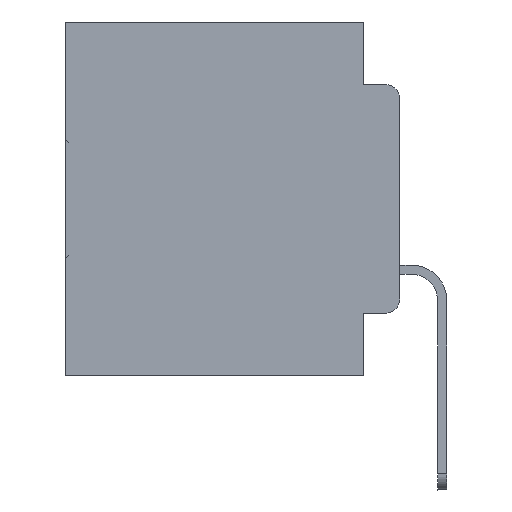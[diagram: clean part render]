
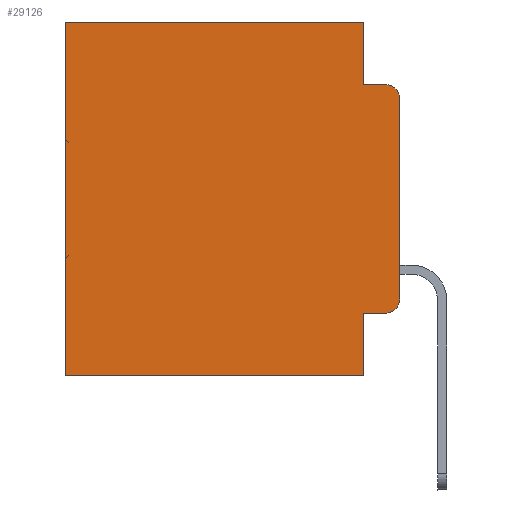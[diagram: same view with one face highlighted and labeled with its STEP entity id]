
A CAD part, left-side view. The second image highlights one B-rep face of the part: STEP entity #29126.
In plain terms, the highlighted planar face has unit normal (-1, 0, 0).
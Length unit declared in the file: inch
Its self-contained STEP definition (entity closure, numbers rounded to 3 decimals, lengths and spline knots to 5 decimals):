
#203 = ORIENTED_EDGE ( 'NONE', *, *, #19037, .F. ) ;
#785 = CARTESIAN_POINT ( 'NONE',  ( 0.298, 0.051, -0.4115 ) ) ;
#797 = CARTESIAN_POINT ( 'NONE',  ( 0.298, 0.051, -0.0885 ) ) ;
#1045 = CARTESIAN_POINT ( 'NONE',  ( 0.298, 0.051, -0.4115 ) ) ;
#1375 = LINE ( 'NONE', #26889, #33483 ) ;
#1922 = VERTEX_POINT ( 'NONE', #797 ) ;
#2664 = CARTESIAN_POINT ( 'NONE',  ( 0.298, 0.02, -0.0885 ) ) ;
#3745 = VECTOR ( 'NONE', #27782, 39.37008 ) ;
#3955 = CARTESIAN_POINT ( 'NONE',  ( 0.298, 0., 0. ) ) ;
#4138 = VECTOR ( 'NONE', #32018, 39.37008 ) ;
#4243 = DIRECTION ( 'NONE',  ( 0., 0., -1. ) ) ;
#4672 = EDGE_CURVE ( 'NONE', #22422, #25049, #24393, .T. ) ;
#5444 = EDGE_CURVE ( 'NONE', #22422, #16145, #26479, .T. ) ;
#6276 = EDGE_CURVE ( 'NONE', #11532, #1922, #30458, .T. ) ;
#6786 = CARTESIAN_POINT ( 'NONE',  ( 0.298, 0.051, 0. ) ) ;
#6876 = LINE ( 'NONE', #11824, #32562 ) ;
#7159 = ORIENTED_EDGE ( 'NONE', *, *, #19411, .F. ) ;
#7215 = LINE ( 'NONE', #12156, #33064 ) ;
#7383 = DIRECTION ( 'NONE',  ( -1., 0., 0. ) ) ;
#7546 = EDGE_CURVE ( 'NONE', #27382, #16145, #22654, .T. ) ;
#9213 = CARTESIAN_POINT ( 'NONE',  ( 0.298, 0.02, -0.1085 ) ) ;
#10151 = VERTEX_POINT ( 'NONE', #33325 ) ;
#10213 = VERTEX_POINT ( 'NONE', #17816 ) ;
#10819 = ORIENTED_EDGE ( 'NONE', *, *, #19772, .T. ) ;
#11026 = EDGE_LOOP ( 'NONE', ( #22251, #27585, #12315, #16645, #33465, #10819, #7159, #203, #27993, #17026 ) ) ;
#11532 = VERTEX_POINT ( 'NONE', #12562 ) ;
#11819 = DIRECTION ( 'NONE',  ( 0., 0., -1. ) ) ;
#11824 = CARTESIAN_POINT ( 'NONE',  ( 0.298, 0., -0.5 ) ) ;
#12156 = CARTESIAN_POINT ( 'NONE',  ( 0.298, 0.051, 0. ) ) ;
#12315 = ORIENTED_EDGE ( 'NONE', *, *, #27359, .F. ) ;
#12464 = CARTESIAN_POINT ( 'NONE',  ( 0.298, 0., -0.1085 ) ) ;
#12562 = CARTESIAN_POINT ( 'NONE',  ( 0.298, 0.051, 0. ) ) ;
#14028 = VECTOR ( 'NONE', #32125, 39.37008 ) ;
#14323 = DIRECTION ( 'NONE',  ( 0., 0., -1. ) ) ;
#15265 = VECTOR ( 'NONE', #32351, 39.37008 ) ;
#15371 = VECTOR ( 'NONE', #4243, 39.37008 ) ;
#16145 = VERTEX_POINT ( 'NONE', #25894 ) ;
#16360 = CARTESIAN_POINT ( 'NONE',  ( 0.298, 0.473, -0.5 ) ) ;
#16645 = ORIENTED_EDGE ( 'NONE', *, *, #6276, .F. ) ;
#16893 = PLANE ( 'NONE',  #33505 ) ;
#17026 = ORIENTED_EDGE ( 'NONE', *, *, #7546, .T. ) ;
#17035 = DIRECTION ( 'NONE',  ( -1., 0., 0. ) ) ;
#17213 = LINE ( 'NONE', #19917, #3745 ) ;
#17608 = CARTESIAN_POINT ( 'NONE',  ( 0.298, 0.02, -0.3915 ) ) ;
#17816 = CARTESIAN_POINT ( 'NONE',  ( 0.298, 0.473, 0. ) ) ;
#19037 = EDGE_CURVE ( 'NONE', #19267, #10151, #7215, .T. ) ;
#19072 = DIRECTION ( 'NONE',  ( 0., 1., 0. ) ) ;
#19267 = VERTEX_POINT ( 'NONE', #785 ) ;
#19411 = EDGE_CURVE ( 'NONE', #10151, #21347, #6876, .T. ) ;
#19772 = EDGE_CURVE ( 'NONE', #10213, #21347, #17213, .T. ) ;
#19917 = CARTESIAN_POINT ( 'NONE',  ( 0.298, 0.473, 0. ) ) ;
#21347 = VERTEX_POINT ( 'NONE', #16360 ) ;
#21455 = DIRECTION ( 'NONE',  ( 1., 0., 0. ) ) ;
#21603 = CARTESIAN_POINT ( 'NONE',  ( 0.298, 0.051, -0.0885 ) ) ;
#21944 = LINE ( 'NONE', #21603, #4138 ) ;
#22251 = ORIENTED_EDGE ( 'NONE', *, *, #5444, .F. ) ;
#22422 = VERTEX_POINT ( 'NONE', #12464 ) ;
#22653 = EDGE_CURVE ( 'NONE', #19267, #27382, #24019, .T. ) ;
#22654 = CIRCLE ( 'NONE', #24814, 0.02 ) ;
#23834 = AXIS2_PLACEMENT_3D ( 'NONE', #9213, #17035, #30305 ) ;
#24019 = LINE ( 'NONE', #1045, #15265 ) ;
#24260 = CARTESIAN_POINT ( 'NONE',  ( 0.298, 0., 0. ) ) ;
#24393 = CIRCLE ( 'NONE', #23834, 0.02 ) ;
#24814 = AXIS2_PLACEMENT_3D ( 'NONE', #17608, #7383, #30392 ) ;
#25049 = VERTEX_POINT ( 'NONE', #2664 ) ;
#25894 = CARTESIAN_POINT ( 'NONE',  ( 0.298, 0., -0.3915 ) ) ;
#26479 = LINE ( 'NONE', #24260, #14028 ) ;
#26757 = FACE_OUTER_BOUND ( 'NONE', #11026, .T. ) ;
#26889 = CARTESIAN_POINT ( 'NONE',  ( 0.298, 0., 0. ) ) ;
#27314 = EDGE_CURVE ( 'NONE', #11532, #10213, #1375, .T. ) ;
#27359 = EDGE_CURVE ( 'NONE', #1922, #25049, #21944, .T. ) ;
#27382 = VERTEX_POINT ( 'NONE', #28910 ) ;
#27585 = ORIENTED_EDGE ( 'NONE', *, *, #4672, .T. ) ;
#27782 = DIRECTION ( 'NONE',  ( 0., 0., -1. ) ) ;
#27993 = ORIENTED_EDGE ( 'NONE', *, *, #22653, .T. ) ;
#28910 = CARTESIAN_POINT ( 'NONE',  ( 0.298, 0.02, -0.4115 ) ) ;
#29126 = ADVANCED_FACE ( 'NONE', ( #26757 ), #16893, .F. ) ;
#30196 = DIRECTION ( 'NONE',  ( 0., 1., 0. ) ) ;
#30305 = DIRECTION ( 'NONE',  ( 0., 0., -1. ) ) ;
#30392 = DIRECTION ( 'NONE',  ( 0., 0., -1. ) ) ;
#30458 = LINE ( 'NONE', #6786, #15371 ) ;
#32018 = DIRECTION ( 'NONE',  ( 0., -1., 0. ) ) ;
#32125 = DIRECTION ( 'NONE',  ( 0., 0., -1. ) ) ;
#32351 = DIRECTION ( 'NONE',  ( 0., -1., 0. ) ) ;
#32562 = VECTOR ( 'NONE', #30196, 39.37008 ) ;
#33064 = VECTOR ( 'NONE', #11819, 39.37008 ) ;
#33325 = CARTESIAN_POINT ( 'NONE',  ( 0.298, 0.051, -0.5 ) ) ;
#33465 = ORIENTED_EDGE ( 'NONE', *, *, #27314, .T. ) ;
#33483 = VECTOR ( 'NONE', #19072, 39.37008 ) ;
#33505 = AXIS2_PLACEMENT_3D ( 'NONE', #3955, #21455, #14323 ) ;
